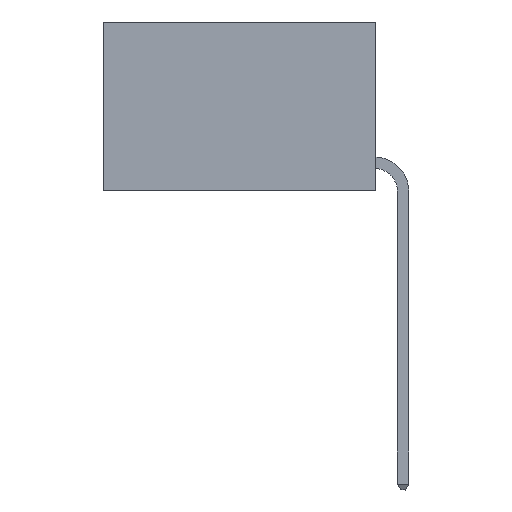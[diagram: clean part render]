
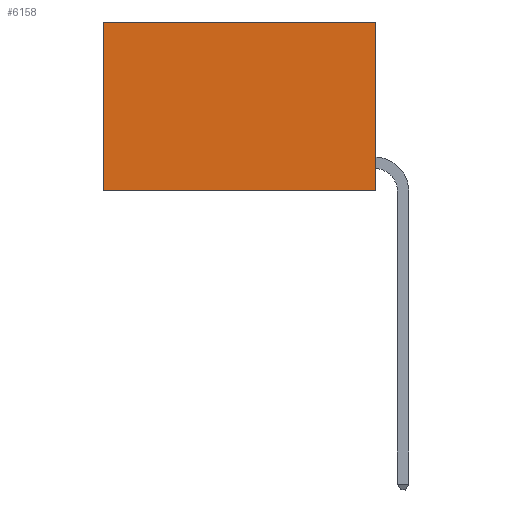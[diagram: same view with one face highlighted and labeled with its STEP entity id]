
A CAD part, left-side view. The second image highlights one B-rep face of the part: STEP entity #6158.
In plain terms, the highlighted planar face has unit normal (-1, 0, 0).
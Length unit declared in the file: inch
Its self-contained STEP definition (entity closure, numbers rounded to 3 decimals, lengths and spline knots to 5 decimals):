
#526 = DIRECTION ( 'NONE',  ( 0., 0., -1. ) ) ;
#600 = ORIENTED_EDGE ( 'NONE', *, *, #16498, .T. ) ;
#2747 = CARTESIAN_POINT ( 'NONE',  ( 0.2625, 0., 0. ) ) ;
#3075 = PLANE ( 'NONE',  #11392 ) ;
#3098 = LINE ( 'NONE', #2747, #10184 ) ;
#3481 = CARTESIAN_POINT ( 'NONE',  ( 0.2625, 0.6, 0. ) ) ;
#3550 = VERTEX_POINT ( 'NONE', #3481 ) ;
#3866 = EDGE_CURVE ( 'NONE', #7263, #10878, #3098, .T. ) ;
#4488 = VECTOR ( 'NONE', #526, 39.37008 ) ;
#4503 = DIRECTION ( 'NONE',  ( 1., 0., 0. ) ) ;
#5056 = ORIENTED_EDGE ( 'NONE', *, *, #7452, .T. ) ;
#5312 = LINE ( 'NONE', #7236, #5762 ) ;
#5762 = VECTOR ( 'NONE', #16925, 39.37008 ) ;
#6158 = ADVANCED_FACE ( 'NONE', ( #14027 ), #3075, .F. ) ;
#6957 = VECTOR ( 'NONE', #17003, 39.37008 ) ;
#7005 = DIRECTION ( 'NONE',  ( 0., 0., -1. ) ) ;
#7192 = EDGE_LOOP ( 'NONE', ( #600, #16491, #17201, #5056 ) ) ;
#7236 = CARTESIAN_POINT ( 'NONE',  ( 0.2625, 0., -0.37 ) ) ;
#7263 = VERTEX_POINT ( 'NONE', #11086 ) ;
#7452 = EDGE_CURVE ( 'NONE', #7263, #3550, #13980, .T. ) ;
#7937 = EDGE_CURVE ( 'NONE', #10878, #16359, #5312, .T. ) ;
#8670 = CARTESIAN_POINT ( 'NONE',  ( 0.2625, 0., 0. ) ) ;
#10184 = VECTOR ( 'NONE', #7005, 39.37008 ) ;
#10878 = VERTEX_POINT ( 'NONE', #14237 ) ;
#11086 = CARTESIAN_POINT ( 'NONE',  ( 0.2625, 0., 0. ) ) ;
#11392 = AXIS2_PLACEMENT_3D ( 'NONE', #12952, #4503, #14336 ) ;
#11559 = LINE ( 'NONE', #17267, #4488 ) ;
#12813 = CARTESIAN_POINT ( 'NONE',  ( 0.2625, 0.6, -0.37 ) ) ;
#12952 = CARTESIAN_POINT ( 'NONE',  ( 0.2625, 0., 0. ) ) ;
#13980 = LINE ( 'NONE', #8670, #6957 ) ;
#14027 = FACE_OUTER_BOUND ( 'NONE', #7192, .T. ) ;
#14237 = CARTESIAN_POINT ( 'NONE',  ( 0.2625, 0., -0.37 ) ) ;
#14336 = DIRECTION ( 'NONE',  ( 0., 0., -1. ) ) ;
#16359 = VERTEX_POINT ( 'NONE', #12813 ) ;
#16491 = ORIENTED_EDGE ( 'NONE', *, *, #7937, .F. ) ;
#16498 = EDGE_CURVE ( 'NONE', #3550, #16359, #11559, .T. ) ;
#16925 = DIRECTION ( 'NONE',  ( 0., 1., 0. ) ) ;
#17003 = DIRECTION ( 'NONE',  ( 0., 1., 0. ) ) ;
#17201 = ORIENTED_EDGE ( 'NONE', *, *, #3866, .F. ) ;
#17267 = CARTESIAN_POINT ( 'NONE',  ( 0.2625, 0.6, 0. ) ) ;
